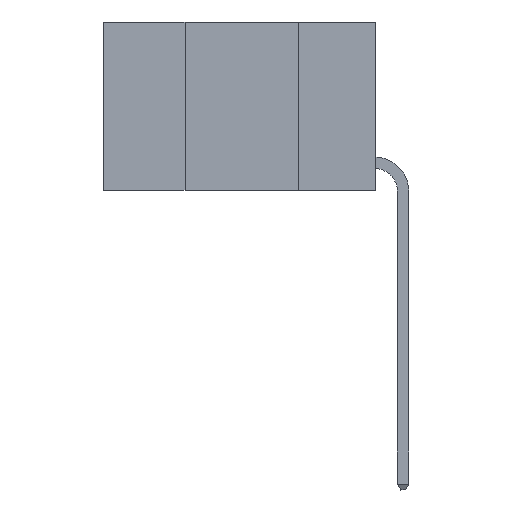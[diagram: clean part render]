
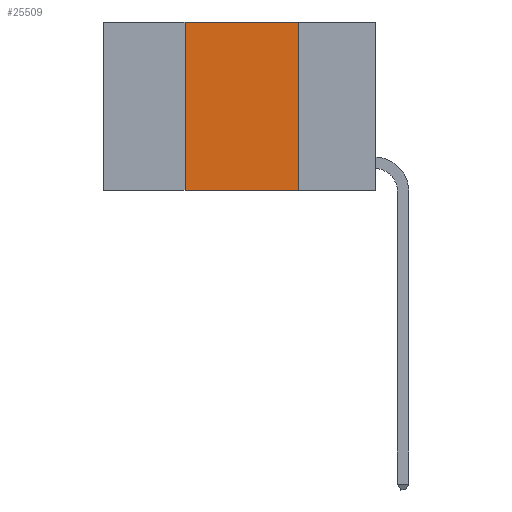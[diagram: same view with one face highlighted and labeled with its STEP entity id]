
A CAD part, left-side view. The second image highlights one B-rep face of the part: STEP entity #25509.
In plain terms, the highlighted planar face has unit normal (-1, 0, 0).
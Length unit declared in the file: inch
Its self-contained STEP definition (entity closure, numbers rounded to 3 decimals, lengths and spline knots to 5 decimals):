
#143 = CARTESIAN_POINT ( 'NONE',  ( 0., 0.17, -0.37 ) ) ;
#1272 = CARTESIAN_POINT ( 'NONE',  ( 0., 0.6, 0. ) ) ;
#1584 = LINE ( 'NONE', #10415, #6933 ) ;
#2779 = VECTOR ( 'NONE', #10711, 39.37008 ) ;
#4867 = EDGE_CURVE ( 'NONE', #14602, #17037, #21124, .T. ) ;
#5775 = CARTESIAN_POINT ( 'NONE',  ( 0., 0.42, -0.37 ) ) ;
#6933 = VECTOR ( 'NONE', #8414, 39.37008 ) ;
#7049 = EDGE_CURVE ( 'NONE', #25378, #14602, #14825, .T. ) ;
#7690 = ORIENTED_EDGE ( 'NONE', *, *, #21668, .T. ) ;
#8250 = CARTESIAN_POINT ( 'NONE',  ( 0., 0.42, 0. ) ) ;
#8414 = DIRECTION ( 'NONE',  ( 0., -1., 0. ) ) ;
#9117 = DIRECTION ( 'NONE',  ( 0., 0., -1. ) ) ;
#10261 = DIRECTION ( 'NONE',  ( 0., -1., 0. ) ) ;
#10285 = AXIS2_PLACEMENT_3D ( 'NONE', #24497, #20117, #9117 ) ;
#10313 = ORIENTED_EDGE ( 'NONE', *, *, #4867, .F. ) ;
#10415 = CARTESIAN_POINT ( 'NONE',  ( 0., 0.6, -0.37 ) ) ;
#10711 = DIRECTION ( 'NONE',  ( 0., 0., -1. ) ) ;
#13059 = ORIENTED_EDGE ( 'NONE', *, *, #7049, .F. ) ;
#13297 = FACE_OUTER_BOUND ( 'NONE', #15815, .T. ) ;
#13320 = VECTOR ( 'NONE', #10261, 39.37008 ) ;
#14602 = VERTEX_POINT ( 'NONE', #8250 ) ;
#14825 = LINE ( 'NONE', #21658, #20740 ) ;
#15815 = EDGE_LOOP ( 'NONE', ( #19762, #10313, #13059, #7690 ) ) ;
#17037 = VERTEX_POINT ( 'NONE', #27693 ) ;
#17316 = DIRECTION ( 'NONE',  ( 0., 0., 1. ) ) ;
#17790 = PLANE ( 'NONE',  #10285 ) ;
#17936 = LINE ( 'NONE', #24644, #2779 ) ;
#19762 = ORIENTED_EDGE ( 'NONE', *, *, #20520, .F. ) ;
#20117 = DIRECTION ( 'NONE',  ( 1., 0., 0. ) ) ;
#20520 = EDGE_CURVE ( 'NONE', #17037, #28035, #17936, .T. ) ;
#20740 = VECTOR ( 'NONE', #17316, 39.37008 ) ;
#21124 = LINE ( 'NONE', #1272, #13320 ) ;
#21658 = CARTESIAN_POINT ( 'NONE',  ( 0., 0.42, 0. ) ) ;
#21668 = EDGE_CURVE ( 'NONE', #25378, #28035, #1584, .T. ) ;
#24497 = CARTESIAN_POINT ( 'NONE',  ( 0., 0.6, 0. ) ) ;
#24644 = CARTESIAN_POINT ( 'NONE',  ( 0., 0.17, 0. ) ) ;
#25378 = VERTEX_POINT ( 'NONE', #5775 ) ;
#25509 = ADVANCED_FACE ( 'NONE', ( #13297 ), #17790, .F. ) ;
#27693 = CARTESIAN_POINT ( 'NONE',  ( 0., 0.17, 0. ) ) ;
#28035 = VERTEX_POINT ( 'NONE', #143 ) ;
